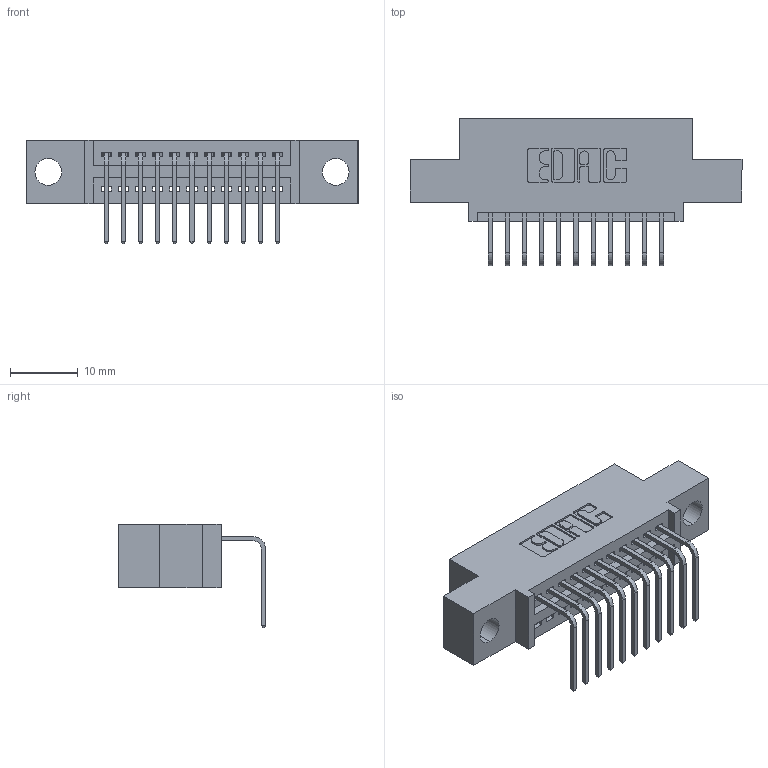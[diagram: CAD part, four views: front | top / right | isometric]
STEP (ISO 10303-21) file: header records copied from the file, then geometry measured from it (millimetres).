
FILE_DESCRIPTION (( 'STEP AP203' ), '1' );
FILE_NAME ('345-011-558-404.STEP', '2021-06-01T16:13:26', ( '' ), ( '' ), 'SwSTEP 2.0', 'SolidWorks 2020', '' );
FILE_SCHEMA (( 'CONFIG_CONTROL_DESIGN' ));
Length unit declared in the file: inch
Products named in the file (3): 345-292-001_558 Tail - 2; 345 Part_0.110 Offset - 0.156 Dia-TI; 345-011-558-404
Assembly tree (12 placements, depth 2):
  345-011-558-404
    345 Part_0.110 Offset - 0.156 Dia-TI
    345-292-001_558 Tail - 2  x11
Bounding box: 49.15 x 21.83 x 15.37 mm (x, y, z)
Volume: 4271.6 mm3; surface area: 5395 mm2
Topology: 12 solids, 12 shells, 804 faces, 2391 edges, 1578 vertices
Faces by surface type: plane 560, cylinder 244
Entity records: 13087 total; most frequent: CARTESIAN_POINT 2279, ORIENTED_EDGE 2222, DIRECTION 2033, EDGE_CURVE 1111, LINE 935, VECTOR 935, VERTEX_POINT 738, AXIS2_PLACEMENT_3D 549
